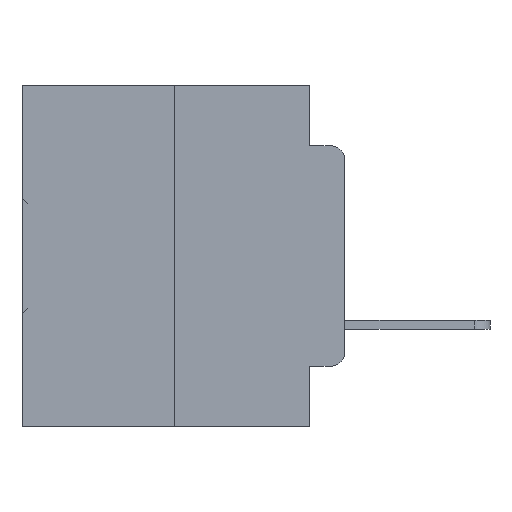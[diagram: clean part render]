
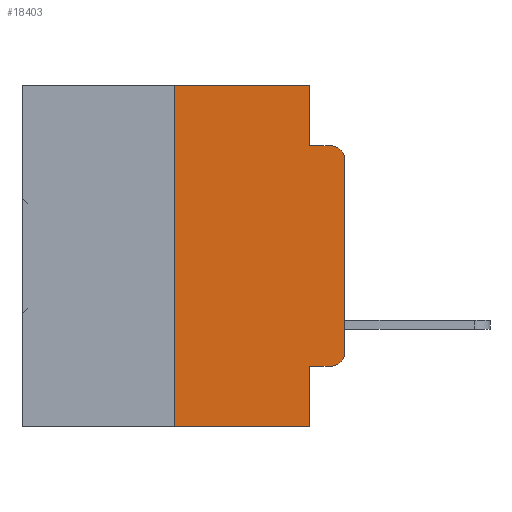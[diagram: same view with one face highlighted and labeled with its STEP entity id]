
A CAD part, left-side view. The second image highlights one B-rep face of the part: STEP entity #18403.
In plain terms, the highlighted planar face has unit normal (-1, 0, 0).
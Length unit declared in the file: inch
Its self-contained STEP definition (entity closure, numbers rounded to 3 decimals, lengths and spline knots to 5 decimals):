
#935 = DIRECTION ( 'NONE',  ( 0., -1., 0. ) ) ;
#1002 = CARTESIAN_POINT ( 'NONE',  ( 0., 0.051, -0.0885 ) ) ;
#1361 = VECTOR ( 'NONE', #11848, 39.37008 ) ;
#1504 = AXIS2_PLACEMENT_3D ( 'NONE', #4199, #23980, #7105 ) ;
#1779 = DIRECTION ( 'NONE',  ( 0., 0., -1. ) ) ;
#1802 = EDGE_CURVE ( 'NONE', #32317, #23822, #15119, .T. ) ;
#2318 = VERTEX_POINT ( 'NONE', #31489 ) ;
#3259 = EDGE_CURVE ( 'NONE', #11704, #3749, #20734, .T. ) ;
#3393 = VERTEX_POINT ( 'NONE', #7021 ) ;
#3749 = VERTEX_POINT ( 'NONE', #11324 ) ;
#3761 = ORIENTED_EDGE ( 'NONE', *, *, #11612, .T. ) ;
#4199 = CARTESIAN_POINT ( 'NONE',  ( 0., 0.02, -0.3915 ) ) ;
#4208 = VERTEX_POINT ( 'NONE', #13156 ) ;
#5355 = LINE ( 'NONE', #13663, #33328 ) ;
#5751 = ORIENTED_EDGE ( 'NONE', *, *, #1802, .F. ) ;
#5811 = EDGE_CURVE ( 'NONE', #4208, #3749, #23459, .T. ) ;
#5920 = EDGE_CURVE ( 'NONE', #26515, #34683, #14232, .T. ) ;
#7021 = CARTESIAN_POINT ( 'NONE',  ( 0., 0., -0.1085 ) ) ;
#7105 = DIRECTION ( 'NONE',  ( 0., 0., -1. ) ) ;
#7448 = VECTOR ( 'NONE', #16379, 39.37008 ) ;
#9078 = CARTESIAN_POINT ( 'NONE',  ( 0., 0.02, -0.0885 ) ) ;
#9632 = DIRECTION ( 'NONE',  ( 0., 0., -1. ) ) ;
#9848 = LINE ( 'NONE', #34054, #1361 ) ;
#11324 = CARTESIAN_POINT ( 'NONE',  ( 0., 0.051, -0.5 ) ) ;
#11412 = LINE ( 'NONE', #32556, #25500 ) ;
#11612 = EDGE_CURVE ( 'NONE', #11704, #26515, #9848, .T. ) ;
#11704 = VERTEX_POINT ( 'NONE', #34506 ) ;
#11848 = DIRECTION ( 'NONE',  ( 0., -1., 0. ) ) ;
#12277 = ORIENTED_EDGE ( 'NONE', *, *, #35553, .T. ) ;
#12517 = CARTESIAN_POINT ( 'NONE',  ( 0., 0.051, -0.0885 ) ) ;
#12563 = ORIENTED_EDGE ( 'NONE', *, *, #5920, .T. ) ;
#13156 = CARTESIAN_POINT ( 'NONE',  ( 0., 0.25, -0.5 ) ) ;
#13437 = AXIS2_PLACEMENT_3D ( 'NONE', #23701, #26507, #9632 ) ;
#13663 = CARTESIAN_POINT ( 'NONE',  ( 0., 0.051, 0. ) ) ;
#14232 = CIRCLE ( 'NONE', #1504, 0.02 ) ;
#14503 = DIRECTION ( 'NONE',  ( -1., 0., 0. ) ) ;
#14565 = DIRECTION ( 'NONE',  ( 0., 0., 1. ) ) ;
#14695 = EDGE_CURVE ( 'NONE', #4208, #2318, #29808, .T. ) ;
#15119 = LINE ( 'NONE', #1002, #21680 ) ;
#15934 = DIRECTION ( 'NONE',  ( 0., -1., 0. ) ) ;
#16379 = DIRECTION ( 'NONE',  ( 0., 0., 1. ) ) ;
#16515 = DIRECTION ( 'NONE',  ( 0., 0., -1. ) ) ;
#16965 = CIRCLE ( 'NONE', #30513, 0.02 ) ;
#18403 = ADVANCED_FACE ( 'NONE', ( #22701 ), #29175, .F. ) ;
#19228 = ORIENTED_EDGE ( 'NONE', *, *, #32422, .F. ) ;
#19510 = CARTESIAN_POINT ( 'NONE',  ( 0., 0.02, -0.4115 ) ) ;
#19527 = ORIENTED_EDGE ( 'NONE', *, *, #5811, .T. ) ;
#20575 = ORIENTED_EDGE ( 'NONE', *, *, #27128, .F. ) ;
#20734 = LINE ( 'NONE', #27228, #28160 ) ;
#21680 = VECTOR ( 'NONE', #26496, 39.37008 ) ;
#22491 = VERTEX_POINT ( 'NONE', #31583 ) ;
#22701 = FACE_OUTER_BOUND ( 'NONE', #35298, .T. ) ;
#23459 = LINE ( 'NONE', #31807, #29956 ) ;
#23701 = CARTESIAN_POINT ( 'NONE',  ( 0., 0.473, 0. ) ) ;
#23822 = VERTEX_POINT ( 'NONE', #9078 ) ;
#23980 = DIRECTION ( 'NONE',  ( -1., 0., 0. ) ) ;
#24815 = VECTOR ( 'NONE', #14565, 39.37008 ) ;
#24863 = CARTESIAN_POINT ( 'NONE',  ( 0., 0.25, 0. ) ) ;
#24969 = ORIENTED_EDGE ( 'NONE', *, *, #29465, .T. ) ;
#25500 = VECTOR ( 'NONE', #15934, 39.37008 ) ;
#25744 = CARTESIAN_POINT ( 'NONE',  ( 0., 0., 0. ) ) ;
#26496 = DIRECTION ( 'NONE',  ( 0., -1., 0. ) ) ;
#26507 = DIRECTION ( 'NONE',  ( 1., 0., 0. ) ) ;
#26515 = VERTEX_POINT ( 'NONE', #19510 ) ;
#27128 = EDGE_CURVE ( 'NONE', #22491, #32317, #5355, .T. ) ;
#27228 = CARTESIAN_POINT ( 'NONE',  ( 0., 0.051, 0. ) ) ;
#27598 = ORIENTED_EDGE ( 'NONE', *, *, #3259, .F. ) ;
#28160 = VECTOR ( 'NONE', #1779, 39.37008 ) ;
#29175 = PLANE ( 'NONE',  #13437 ) ;
#29237 = ORIENTED_EDGE ( 'NONE', *, *, #14695, .F. ) ;
#29465 = EDGE_CURVE ( 'NONE', #34683, #3393, #32086, .T. ) ;
#29808 = LINE ( 'NONE', #24863, #7448 ) ;
#29956 = VECTOR ( 'NONE', #935, 39.37008 ) ;
#30513 = AXIS2_PLACEMENT_3D ( 'NONE', #31194, #14503, #33896 ) ;
#31194 = CARTESIAN_POINT ( 'NONE',  ( 0., 0.02, -0.1085 ) ) ;
#31489 = CARTESIAN_POINT ( 'NONE',  ( 0., 0.25, 0. ) ) ;
#31583 = CARTESIAN_POINT ( 'NONE',  ( 0., 0.051, 0. ) ) ;
#31807 = CARTESIAN_POINT ( 'NONE',  ( 0., 0.473, -0.5 ) ) ;
#32086 = LINE ( 'NONE', #25744, #24815 ) ;
#32317 = VERTEX_POINT ( 'NONE', #12517 ) ;
#32422 = EDGE_CURVE ( 'NONE', #2318, #22491, #11412, .T. ) ;
#32556 = CARTESIAN_POINT ( 'NONE',  ( 0., 0.473, 0. ) ) ;
#33328 = VECTOR ( 'NONE', #16515, 39.37008 ) ;
#33896 = DIRECTION ( 'NONE',  ( 0., 0., -1. ) ) ;
#34054 = CARTESIAN_POINT ( 'NONE',  ( 0., 0.051, -0.4115 ) ) ;
#34506 = CARTESIAN_POINT ( 'NONE',  ( 0., 0.051, -0.4115 ) ) ;
#34683 = VERTEX_POINT ( 'NONE', #34748 ) ;
#34748 = CARTESIAN_POINT ( 'NONE',  ( 0., 0., -0.3915 ) ) ;
#35298 = EDGE_LOOP ( 'NONE', ( #24969, #12277, #5751, #20575, #19228, #29237, #19527, #27598, #3761, #12563 ) ) ;
#35553 = EDGE_CURVE ( 'NONE', #3393, #23822, #16965, .T. ) ;
